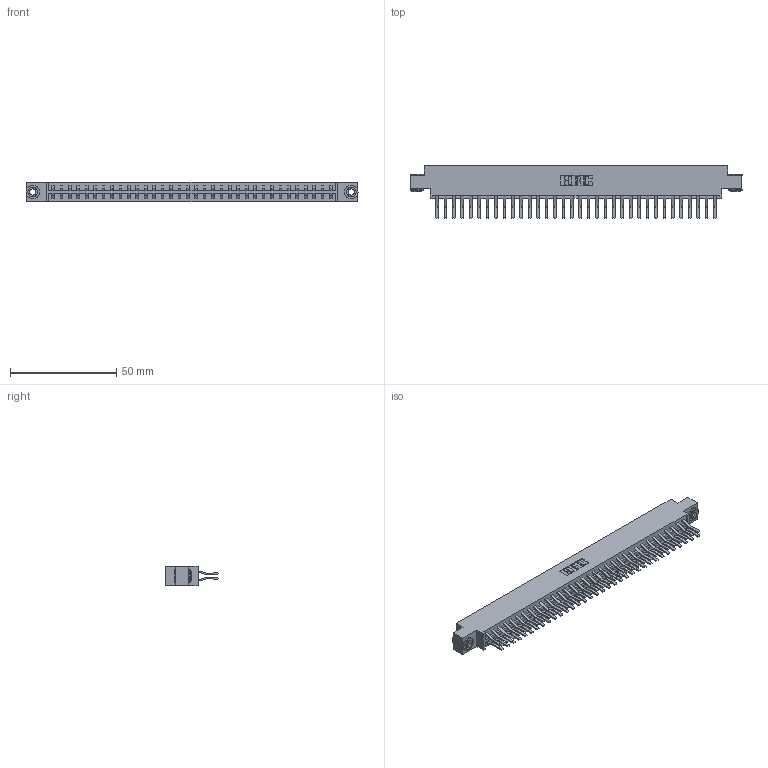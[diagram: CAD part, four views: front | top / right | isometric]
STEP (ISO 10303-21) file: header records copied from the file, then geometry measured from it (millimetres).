
FILE_DESCRIPTION (( 'STEP AP203' ), '1' );
FILE_NAME ('333-068-560-803.STEP', '2018-08-04T13:58:47', ( '' ), ( '' ), 'SwSTEP 2.0', 'SolidWorks 2016', '' );
FILE_SCHEMA (( 'CONFIG_CONTROL_DESIGN' ));
Length unit declared in the file: inch
Products named in the file (4): 345-250-002_345-250-002-102; 333-068-560-803; 333 Part_Offset - .156 Dia - TH; 345-292-001_560 Tail
Assembly tree (71 placements, depth 2):
  333-068-560-803
    333 Part_Offset - .156 Dia - TH
    345-292-001_560 Tail  x68
    345-250-002_345-250-002-102  x2
Bounding box: 156.26 x 24.78 x 9.4 mm (x, y, z)
Volume: 16115.8 mm3; surface area: 20680.2 mm2
Topology: 71 solids, 71 shells, 3828 faces, 11347 edges, 7470 vertices
Faces by surface type: plane 2532, cylinder 1288, cone 8
Entity records: 23778 total; most frequent: CARTESIAN_POINT 3929, ORIENTED_EDGE 3858, DIRECTION 3407, EDGE_CURVE 1929, LINE 1773, VECTOR 1773, VERTEX_POINT 1282, AXIS2_PLACEMENT_3D 817
